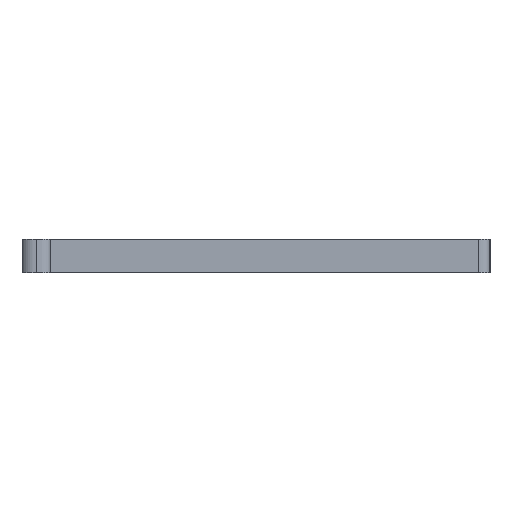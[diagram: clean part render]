
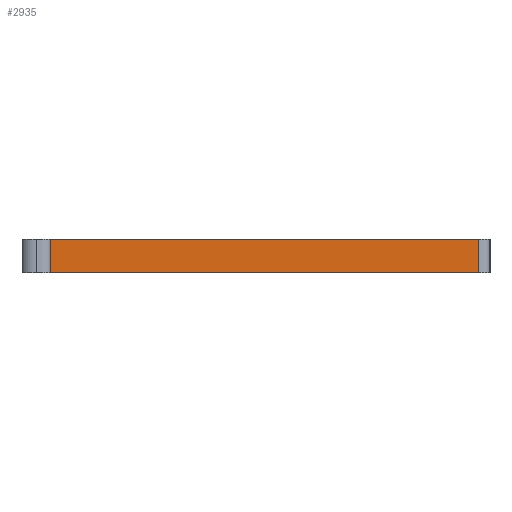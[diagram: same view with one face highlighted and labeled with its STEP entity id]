
A CAD part, left-side view. The second image highlights one B-rep face of the part: STEP entity #2935.
In plain terms, the highlighted planar face has unit normal (-1, 0, 0).
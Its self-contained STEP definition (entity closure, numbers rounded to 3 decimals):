
#97 = EDGE_LOOP ( 'NONE', ( #3617, #2232, #3143, #2301 ) ) ;
#254 = CARTESIAN_POINT ( 'NONE',  ( 135.592, -8.853, 0.203 ) ) ;
#292 = CARTESIAN_POINT ( 'NONE',  ( 135.592, -8.853, 0.203 ) ) ;
#307 = CARTESIAN_POINT ( 'NONE',  ( 135.592, -8.853, 0.203 ) ) ;
#322 = DIRECTION ( 'NONE',  ( 0., -1., 0. ) ) ;
#983 = DIRECTION ( 'NONE',  ( 0., 0., -1. ) ) ;
#1049 = VECTOR ( 'NONE', #322, 1000. ) ;
#1104 = LINE ( 'NONE', #292, #1049 ) ;
#1233 = CARTESIAN_POINT ( 'NONE',  ( 135.592, -11.437, 0.203 ) ) ;
#1773 = DIRECTION ( 'NONE',  ( 0., 0., -1. ) ) ;
#2179 = DIRECTION ( 'NONE',  ( 0., 0., -1. ) ) ;
#2197 = CARTESIAN_POINT ( 'NONE',  ( 135.592, -8.853, 0.203 ) ) ;
#2219 = PLANE ( 'NONE',  #3910 ) ;
#2229 = CARTESIAN_POINT ( 'NONE',  ( 135.592, -11.437, 0.203 ) ) ;
#2232 = ORIENTED_EDGE ( 'NONE', *, *, #5859, .F. ) ;
#2259 = CARTESIAN_POINT ( 'NONE',  ( 135.592, -8.853, 0. ) ) ;
#2261 = VECTOR ( 'NONE', #5267, 1000. ) ;
#2301 = ORIENTED_EDGE ( 'NONE', *, *, #5511, .T. ) ;
#2319 = DIRECTION ( 'NONE',  ( 1., 0., 0. ) ) ;
#2338 = LINE ( 'NONE', #6169, #2261 ) ;
#2555 = LINE ( 'NONE', #1233, #6340 ) ;
#2874 = FACE_OUTER_BOUND ( 'NONE', #97, .T. ) ;
#2935 = ADVANCED_FACE ( 'NONE', ( #2874 ), #2219, .F. ) ;
#3143 = ORIENTED_EDGE ( 'NONE', *, *, #6194, .F. ) ;
#3542 = VERTEX_POINT ( 'NONE', #307 ) ;
#3580 = VECTOR ( 'NONE', #983, 1000. ) ;
#3617 = ORIENTED_EDGE ( 'NONE', *, *, #5962, .T. ) ;
#3712 = LINE ( 'NONE', #254, #3580 ) ;
#3910 = AXIS2_PLACEMENT_3D ( 'NONE', #2197, #2319, #2179 ) ;
#3952 = VERTEX_POINT ( 'NONE', #5510 ) ;
#4304 = VERTEX_POINT ( 'NONE', #2229 ) ;
#5267 = DIRECTION ( 'NONE',  ( 0., -1., 0. ) ) ;
#5510 = CARTESIAN_POINT ( 'NONE',  ( 135.592, -11.437, 0. ) ) ;
#5511 = EDGE_CURVE ( 'NONE', #3542, #5645, #3712, .T. ) ;
#5645 = VERTEX_POINT ( 'NONE', #2259 ) ;
#5859 = EDGE_CURVE ( 'NONE', #4304, #3952, #2555, .T. ) ;
#5962 = EDGE_CURVE ( 'NONE', #5645, #3952, #2338, .T. ) ;
#6169 = CARTESIAN_POINT ( 'NONE',  ( 135.592, -8.853, 0. ) ) ;
#6194 = EDGE_CURVE ( 'NONE', #3542, #4304, #1104, .T. ) ;
#6340 = VECTOR ( 'NONE', #1773, 1000. ) ;
